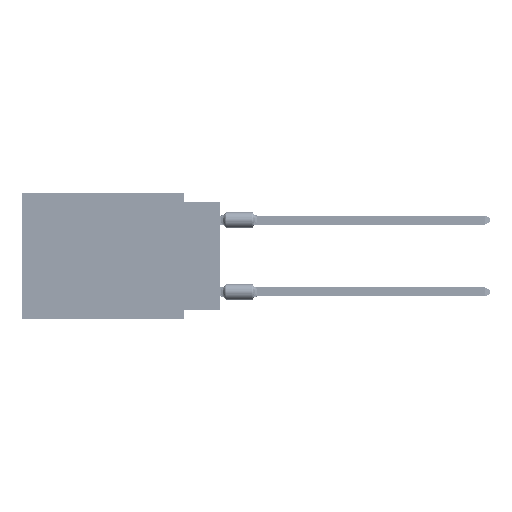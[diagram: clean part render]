
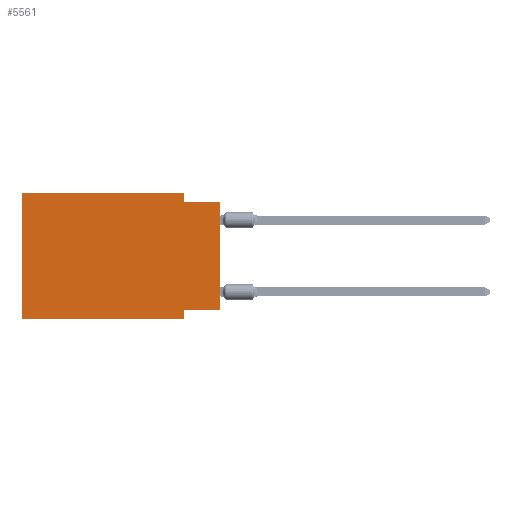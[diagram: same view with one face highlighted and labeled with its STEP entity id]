
A CAD part, left-side view. The second image highlights one B-rep face of the part: STEP entity #5561.
In plain terms, the highlighted planar face has unit normal (-1, 0, 0).
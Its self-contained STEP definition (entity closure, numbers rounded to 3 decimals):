
#275 = LINE ( 'NONE', #62504, #14044 ) ;
#533 = EDGE_CURVE ( 'NONE', #21532, #65815, #9547, .T. ) ;
#938 = VECTOR ( 'NONE', #25244, 1000. ) ;
#2210 = DIRECTION ( 'NONE',  ( 0., 0., 1. ) ) ;
#2949 = VERTEX_POINT ( 'NONE', #22335 ) ;
#5415 = DIRECTION ( 'NONE',  ( 0., -1., 0. ) ) ;
#5561 = ADVANCED_FACE ( 'NONE', ( #11676 ), #36288, .F. ) ;
#5869 = CARTESIAN_POINT ( 'NONE',  ( 0., 13.97, 0. ) ) ;
#6399 = EDGE_CURVE ( 'NONE', #28437, #2949, #9823, .T. ) ;
#9129 = VERTEX_POINT ( 'NONE', #30907 ) ;
#9171 = VECTOR ( 'NONE', #16564, 1000. ) ;
#9538 = DIRECTION ( 'NONE',  ( 0., -1., 0. ) ) ;
#9547 = LINE ( 'NONE', #20116, #938 ) ;
#9823 = LINE ( 'NONE', #42625, #28717 ) ;
#9905 = CARTESIAN_POINT ( 'NONE',  ( 0., 2.54, -0.635 ) ) ;
#10871 = CARTESIAN_POINT ( 'NONE',  ( 0., 0., -0.635 ) ) ;
#11036 = DIRECTION ( 'NONE',  ( 0., 0., -1. ) ) ;
#11676 = FACE_OUTER_BOUND ( 'NONE', #22936, .T. ) ;
#12005 = EDGE_CURVE ( 'NONE', #65815, #27383, #275, .T. ) ;
#13234 = CARTESIAN_POINT ( 'NONE',  ( 0., 13.97, 0. ) ) ;
#14044 = VECTOR ( 'NONE', #9538, 1000. ) ;
#15091 = CARTESIAN_POINT ( 'NONE',  ( 0., 0., -8.255 ) ) ;
#16178 = CARTESIAN_POINT ( 'NONE',  ( 0., 2.54, 0. ) ) ;
#16564 = DIRECTION ( 'NONE',  ( 0., -1., 0. ) ) ;
#19761 = ORIENTED_EDGE ( 'NONE', *, *, #533, .F. ) ;
#20116 = CARTESIAN_POINT ( 'NONE',  ( 0., 13.97, 0. ) ) ;
#21532 = VERTEX_POINT ( 'NONE', #22635 ) ;
#22301 = LINE ( 'NONE', #16178, #61760 ) ;
#22335 = CARTESIAN_POINT ( 'NONE',  ( 0., 2.54, -8.255 ) ) ;
#22635 = CARTESIAN_POINT ( 'NONE',  ( 0., 13.97, -8.89 ) ) ;
#22936 = EDGE_LOOP ( 'NONE', ( #39342, #37055, #37828, #41361, #19761, #38253, #31732, #49123 ) ) ;
#25084 = EDGE_CURVE ( 'NONE', #2949, #9129, #63663, .T. ) ;
#25244 = DIRECTION ( 'NONE',  ( 0., 0., 1. ) ) ;
#27165 = CARTESIAN_POINT ( 'NONE',  ( 0., 0., 0. ) ) ;
#27377 = DIRECTION ( 'NONE',  ( 0., 0., -1. ) ) ;
#27383 = VERTEX_POINT ( 'NONE', #64860 ) ;
#27742 = VECTOR ( 'NONE', #5415, 1000. ) ;
#28437 = VERTEX_POINT ( 'NONE', #15091 ) ;
#28717 = VECTOR ( 'NONE', #46412, 1000. ) ;
#30033 = VECTOR ( 'NONE', #2210, 1000. ) ;
#30907 = CARTESIAN_POINT ( 'NONE',  ( 0., 2.54, -8.89 ) ) ;
#31732 = ORIENTED_EDGE ( 'NONE', *, *, #25084, .F. ) ;
#33483 = EDGE_CURVE ( 'NONE', #21532, #9129, #59206, .T. ) ;
#34767 = EDGE_CURVE ( 'NONE', #28437, #58776, #59301, .T. ) ;
#36288 = PLANE ( 'NONE',  #39562 ) ;
#37055 = ORIENTED_EDGE ( 'NONE', *, *, #63114, .F. ) ;
#37337 = DIRECTION ( 'NONE',  ( 0., 0., -1. ) ) ;
#37828 = ORIENTED_EDGE ( 'NONE', *, *, #49211, .F. ) ;
#38253 = ORIENTED_EDGE ( 'NONE', *, *, #33483, .T. ) ;
#39342 = ORIENTED_EDGE ( 'NONE', *, *, #34767, .T. ) ;
#39562 = AXIS2_PLACEMENT_3D ( 'NONE', #5869, #58514, #27377 ) ;
#40140 = CARTESIAN_POINT ( 'NONE',  ( 0., 0., -0.635 ) ) ;
#41201 = VECTOR ( 'NONE', #37337, 1000. ) ;
#41361 = ORIENTED_EDGE ( 'NONE', *, *, #12005, .F. ) ;
#42625 = CARTESIAN_POINT ( 'NONE',  ( 0., 0., -8.255 ) ) ;
#46412 = DIRECTION ( 'NONE',  ( 0., 1., 0. ) ) ;
#49123 = ORIENTED_EDGE ( 'NONE', *, *, #6399, .F. ) ;
#49211 = EDGE_CURVE ( 'NONE', #27383, #59113, #22301, .T. ) ;
#52928 = LINE ( 'NONE', #10871, #27742 ) ;
#54434 = CARTESIAN_POINT ( 'NONE',  ( 0., 2.54, -8.89 ) ) ;
#54746 = CARTESIAN_POINT ( 'NONE',  ( 0., 13.97, -8.89 ) ) ;
#58514 = DIRECTION ( 'NONE',  ( 1., 0., 0. ) ) ;
#58776 = VERTEX_POINT ( 'NONE', #40140 ) ;
#59113 = VERTEX_POINT ( 'NONE', #9905 ) ;
#59206 = LINE ( 'NONE', #54746, #9171 ) ;
#59301 = LINE ( 'NONE', #27165, #30033 ) ;
#61760 = VECTOR ( 'NONE', #11036, 1000. ) ;
#62504 = CARTESIAN_POINT ( 'NONE',  ( 0., 13.97, 0. ) ) ;
#63114 = EDGE_CURVE ( 'NONE', #59113, #58776, #52928, .T. ) ;
#63663 = LINE ( 'NONE', #54434, #41201 ) ;
#64860 = CARTESIAN_POINT ( 'NONE',  ( 0., 2.54, 0. ) ) ;
#65815 = VERTEX_POINT ( 'NONE', #13234 ) ;
